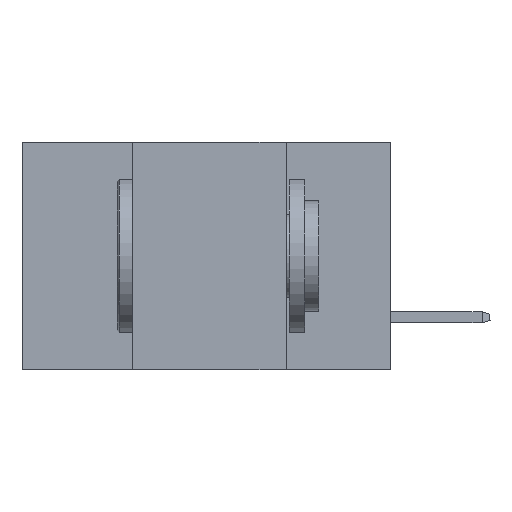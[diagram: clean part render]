
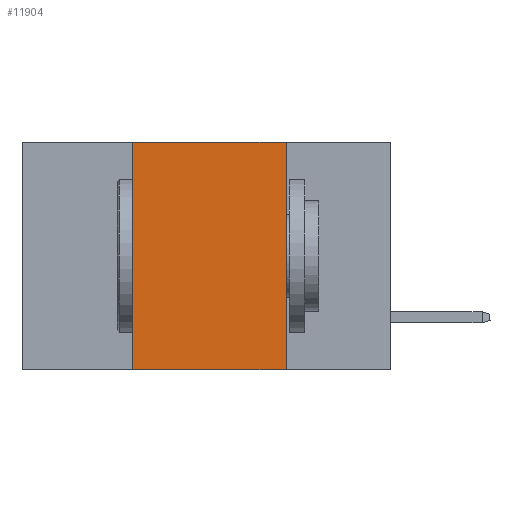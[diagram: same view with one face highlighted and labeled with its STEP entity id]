
A CAD part, left-side view. The second image highlights one B-rep face of the part: STEP entity #11904.
In plain terms, the highlighted planar face has unit normal (-1, 0, 0).
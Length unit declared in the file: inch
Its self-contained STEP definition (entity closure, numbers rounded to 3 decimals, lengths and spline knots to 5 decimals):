
#547 = CARTESIAN_POINT ( 'NONE',  ( 0., 0.17, 0. ) ) ;
#1229 = CARTESIAN_POINT ( 'NONE',  ( 0., 0.17, 0. ) ) ;
#1676 = VERTEX_POINT ( 'NONE', #1738 ) ;
#1738 = CARTESIAN_POINT ( 'NONE',  ( 0., 0.17, -0.37 ) ) ;
#1869 = DIRECTION ( 'NONE',  ( 0., 0., 1. ) ) ;
#2006 = CARTESIAN_POINT ( 'NONE',  ( 0., 0.6, 0. ) ) ;
#2282 = EDGE_CURVE ( 'NONE', #3924, #6400, #6977, .T. ) ;
#2375 = CARTESIAN_POINT ( 'NONE',  ( 0., 0.42, 0. ) ) ;
#2825 = EDGE_CURVE ( 'NONE', #3924, #1676, #7166, .T. ) ;
#3277 = CARTESIAN_POINT ( 'NONE',  ( 0., 0.6, 0. ) ) ;
#3337 = DIRECTION ( 'NONE',  ( 0., 0., -1. ) ) ;
#3793 = EDGE_CURVE ( 'NONE', #8636, #1676, #4575, .T. ) ;
#3924 = VERTEX_POINT ( 'NONE', #5210 ) ;
#4484 = CARTESIAN_POINT ( 'NONE',  ( 0., 0.42, 0. ) ) ;
#4514 = LINE ( 'NONE', #2006, #16364 ) ;
#4575 = LINE ( 'NONE', #1229, #10904 ) ;
#5210 = CARTESIAN_POINT ( 'NONE',  ( 0., 0.42, -0.37 ) ) ;
#6400 = VERTEX_POINT ( 'NONE', #2375 ) ;
#6977 = LINE ( 'NONE', #4484, #8756 ) ;
#7014 = DIRECTION ( 'NONE',  ( 0., -1., 0. ) ) ;
#7166 = LINE ( 'NONE', #10603, #12288 ) ;
#8278 = EDGE_LOOP ( 'NONE', ( #11287, #12015, #10232, #9245 ) ) ;
#8407 = PLANE ( 'NONE',  #12273 ) ;
#8636 = VERTEX_POINT ( 'NONE', #547 ) ;
#8756 = VECTOR ( 'NONE', #1869, 39.37008 ) ;
#9245 = ORIENTED_EDGE ( 'NONE', *, *, #2825, .T. ) ;
#9806 = DIRECTION ( 'NONE',  ( 1., 0., 0. ) ) ;
#10232 = ORIENTED_EDGE ( 'NONE', *, *, #2282, .F. ) ;
#10603 = CARTESIAN_POINT ( 'NONE',  ( 0., 0.6, -0.37 ) ) ;
#10904 = VECTOR ( 'NONE', #15147, 39.37008 ) ;
#11287 = ORIENTED_EDGE ( 'NONE', *, *, #3793, .F. ) ;
#11904 = ADVANCED_FACE ( 'NONE', ( #14580 ), #8407, .F. ) ;
#12015 = ORIENTED_EDGE ( 'NONE', *, *, #13328, .F. ) ;
#12157 = DIRECTION ( 'NONE',  ( 0., -1., 0. ) ) ;
#12273 = AXIS2_PLACEMENT_3D ( 'NONE', #3277, #9806, #3337 ) ;
#12288 = VECTOR ( 'NONE', #7014, 39.37008 ) ;
#13328 = EDGE_CURVE ( 'NONE', #6400, #8636, #4514, .T. ) ;
#14580 = FACE_OUTER_BOUND ( 'NONE', #8278, .T. ) ;
#15147 = DIRECTION ( 'NONE',  ( 0., 0., -1. ) ) ;
#16364 = VECTOR ( 'NONE', #12157, 39.37008 ) ;
